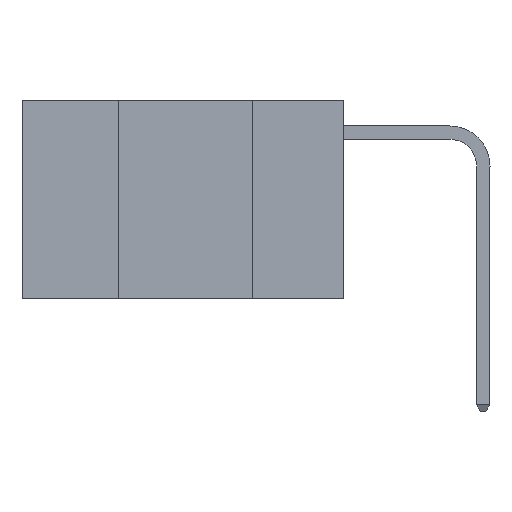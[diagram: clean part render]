
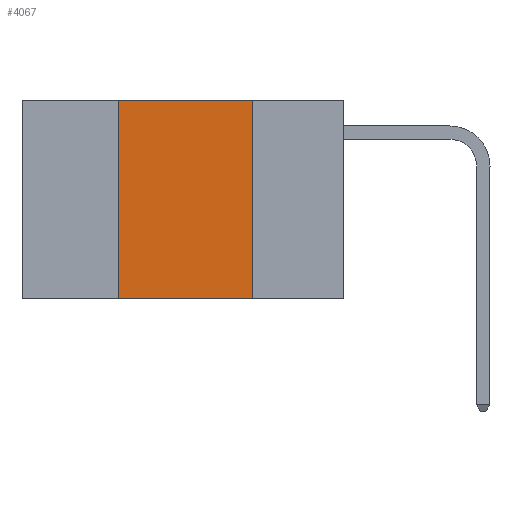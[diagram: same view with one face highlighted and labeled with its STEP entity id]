
A CAD part, left-side view. The second image highlights one B-rep face of the part: STEP entity #4067.
In plain terms, the highlighted planar face has unit normal (-1, 0, 0).
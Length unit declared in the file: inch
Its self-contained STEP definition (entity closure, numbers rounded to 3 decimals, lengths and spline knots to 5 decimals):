
#51 = VECTOR ( 'NONE', #6644, 39.37008 ) ;
#780 = VECTOR ( 'NONE', #2929, 39.37008 ) ;
#970 = CARTESIAN_POINT ( 'NONE',  ( 0., 0.6, -0.37 ) ) ;
#1165 = CARTESIAN_POINT ( 'NONE',  ( 0., 0.6, 0. ) ) ;
#1620 = CARTESIAN_POINT ( 'NONE',  ( 0., 0.17, 0. ) ) ;
#2005 = AXIS2_PLACEMENT_3D ( 'NONE', #8890, #4283, #10715 ) ;
#2095 = DIRECTION ( 'NONE',  ( 0., -1., 0. ) ) ;
#2787 = CARTESIAN_POINT ( 'NONE',  ( 0., 0.42, -0.37 ) ) ;
#2859 = VERTEX_POINT ( 'NONE', #10822 ) ;
#2929 = DIRECTION ( 'NONE',  ( 0., 0., -1. ) ) ;
#4067 = ADVANCED_FACE ( 'NONE', ( #6186 ), #9812, .F. ) ;
#4111 = VECTOR ( 'NONE', #8341, 39.37008 ) ;
#4283 = DIRECTION ( 'NONE',  ( 1., 0., 0. ) ) ;
#4833 = LINE ( 'NONE', #1165, #7005 ) ;
#4940 = ORIENTED_EDGE ( 'NONE', *, *, #9910, .F. ) ;
#5664 = CARTESIAN_POINT ( 'NONE',  ( 0., 0.17, 0. ) ) ;
#5720 = CARTESIAN_POINT ( 'NONE',  ( 0., 0.42, 0. ) ) ;
#6186 = FACE_OUTER_BOUND ( 'NONE', #7406, .T. ) ;
#6294 = LINE ( 'NONE', #970, #4111 ) ;
#6644 = DIRECTION ( 'NONE',  ( 0., 0., 1. ) ) ;
#6756 = VERTEX_POINT ( 'NONE', #2787 ) ;
#7005 = VECTOR ( 'NONE', #2095, 39.37008 ) ;
#7406 = EDGE_LOOP ( 'NONE', ( #4940, #9861, #7681, #10132 ) ) ;
#7409 = LINE ( 'NONE', #5720, #51 ) ;
#7436 = EDGE_CURVE ( 'NONE', #6756, #10501, #6294, .T. ) ;
#7501 = CARTESIAN_POINT ( 'NONE',  ( 0., 0.17, -0.37 ) ) ;
#7585 = EDGE_CURVE ( 'NONE', #2859, #11496, #4833, .T. ) ;
#7681 = ORIENTED_EDGE ( 'NONE', *, *, #9295, .F. ) ;
#7824 = LINE ( 'NONE', #5664, #780 ) ;
#8341 = DIRECTION ( 'NONE',  ( 0., -1., 0. ) ) ;
#8890 = CARTESIAN_POINT ( 'NONE',  ( 0., 0.6, 0. ) ) ;
#9295 = EDGE_CURVE ( 'NONE', #6756, #2859, #7409, .T. ) ;
#9812 = PLANE ( 'NONE',  #2005 ) ;
#9861 = ORIENTED_EDGE ( 'NONE', *, *, #7585, .F. ) ;
#9910 = EDGE_CURVE ( 'NONE', #11496, #10501, #7824, .T. ) ;
#10132 = ORIENTED_EDGE ( 'NONE', *, *, #7436, .T. ) ;
#10501 = VERTEX_POINT ( 'NONE', #7501 ) ;
#10715 = DIRECTION ( 'NONE',  ( 0., 0., -1. ) ) ;
#10822 = CARTESIAN_POINT ( 'NONE',  ( 0., 0.42, 0. ) ) ;
#11496 = VERTEX_POINT ( 'NONE', #1620 ) ;
